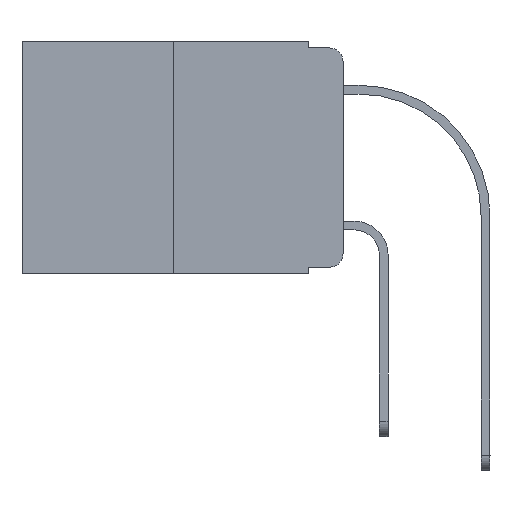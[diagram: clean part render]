
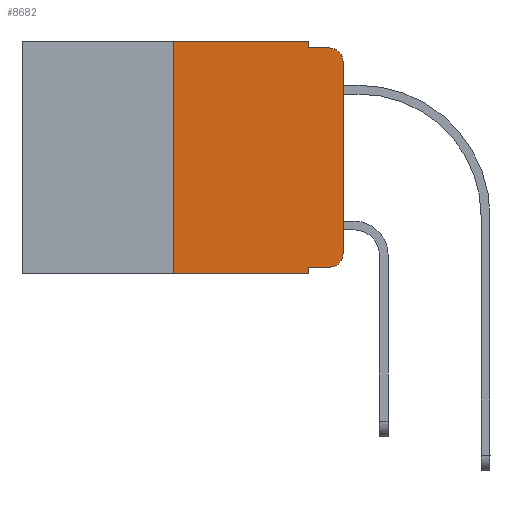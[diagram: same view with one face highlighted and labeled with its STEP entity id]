
A CAD part, left-side view. The second image highlights one B-rep face of the part: STEP entity #8682.
In plain terms, the highlighted planar face has unit normal (-1, 0, 0).
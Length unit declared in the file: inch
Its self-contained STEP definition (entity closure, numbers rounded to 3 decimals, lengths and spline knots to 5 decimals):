
#50 = AXIS2_PLACEMENT_3D ( 'NONE', #10826, #472, #3519 ) ;
#267 = CARTESIAN_POINT ( 'NONE',  ( 0., 0.051, -0.333 ) ) ;
#313 = LINE ( 'NONE', #8908, #887 ) ;
#472 = DIRECTION ( 'NONE',  ( -1., 0., 0. ) ) ;
#727 = ORIENTED_EDGE ( 'NONE', *, *, #12089, .T. ) ;
#887 = VECTOR ( 'NONE', #5989, 39.37008 ) ;
#927 = VERTEX_POINT ( 'NONE', #12649 ) ;
#1011 = DIRECTION ( 'NONE',  ( 0., -1., 0. ) ) ;
#1066 = EDGE_LOOP ( 'NONE', ( #11699, #17623, #16235, #14719, #14676, #9223, #13235, #10024, #4918, #727 ) ) ;
#1161 = DIRECTION ( 'NONE',  ( 0., 0., 1. ) ) ;
#1207 = CIRCLE ( 'NONE', #12118, 0.02 ) ;
#1304 = VERTEX_POINT ( 'NONE', #11146 ) ;
#1893 = VERTEX_POINT ( 'NONE', #14709 ) ;
#2257 = EDGE_CURVE ( 'NONE', #16215, #1304, #1207, .T. ) ;
#2621 = LINE ( 'NONE', #8669, #13465 ) ;
#2675 = LINE ( 'NONE', #18884, #6935 ) ;
#2961 = CARTESIAN_POINT ( 'NONE',  ( 0., 0.473, 0. ) ) ;
#3015 = LINE ( 'NONE', #267, #4621 ) ;
#3328 = DIRECTION ( 'NONE',  ( 0., 0., -1. ) ) ;
#3519 = DIRECTION ( 'NONE',  ( 0., 0., -1. ) ) ;
#3667 = EDGE_CURVE ( 'NONE', #16139, #12094, #17887, .T. ) ;
#4338 = CARTESIAN_POINT ( 'NONE',  ( 0., 0., 0. ) ) ;
#4597 = CARTESIAN_POINT ( 'NONE',  ( 0., 0.02, -0.03 ) ) ;
#4621 = VECTOR ( 'NONE', #16482, 39.37008 ) ;
#4918 = ORIENTED_EDGE ( 'NONE', *, *, #7769, .T. ) ;
#5019 = VERTEX_POINT ( 'NONE', #17820 ) ;
#5074 = CARTESIAN_POINT ( 'NONE',  ( 0., 0.051, 0. ) ) ;
#5329 = VECTOR ( 'NONE', #7359, 39.37008 ) ;
#5377 = CARTESIAN_POINT ( 'NONE',  ( 0., 0.25, 0. ) ) ;
#5652 = DIRECTION ( 'NONE',  ( 0., -1., 0. ) ) ;
#5989 = DIRECTION ( 'NONE',  ( 0., -1., 0. ) ) ;
#6250 = DIRECTION ( 'NONE',  ( 0., 0., -1. ) ) ;
#6935 = VECTOR ( 'NONE', #1011, 39.37008 ) ;
#7359 = DIRECTION ( 'NONE',  ( 0., 0., 1. ) ) ;
#7623 = DIRECTION ( 'NONE',  ( -1., 0., 0. ) ) ;
#7769 = EDGE_CURVE ( 'NONE', #17318, #11249, #3015, .T. ) ;
#8669 = CARTESIAN_POINT ( 'NONE',  ( 0., 0.473, 0. ) ) ;
#8682 = ADVANCED_FACE ( 'NONE', ( #17999 ), #16243, .F. ) ;
#8725 = EDGE_CURVE ( 'NONE', #12094, #1304, #313, .T. ) ;
#8908 = CARTESIAN_POINT ( 'NONE',  ( 0., 0.051, -0.01 ) ) ;
#9108 = DIRECTION ( 'NONE',  ( 0., 0., -1. ) ) ;
#9223 = ORIENTED_EDGE ( 'NONE', *, *, #10721, .F. ) ;
#9567 = LINE ( 'NONE', #5074, #11299 ) ;
#9822 = VERTEX_POINT ( 'NONE', #14780 ) ;
#10024 = ORIENTED_EDGE ( 'NONE', *, *, #12182, .F. ) ;
#10446 = DIRECTION ( 'NONE',  ( 0., 0., -1. ) ) ;
#10721 = EDGE_CURVE ( 'NONE', #9822, #1893, #14545, .T. ) ;
#10826 = CARTESIAN_POINT ( 'NONE',  ( 0., 0.02, -0.313 ) ) ;
#11093 = CARTESIAN_POINT ( 'NONE',  ( 0., 0., -0.03 ) ) ;
#11146 = CARTESIAN_POINT ( 'NONE',  ( 0., 0.02, -0.01 ) ) ;
#11179 = AXIS2_PLACEMENT_3D ( 'NONE', #2961, #11851, #9108 ) ;
#11249 = VERTEX_POINT ( 'NONE', #18303 ) ;
#11299 = VECTOR ( 'NONE', #6250, 39.37008 ) ;
#11387 = EDGE_CURVE ( 'NONE', #9822, #927, #2675, .T. ) ;
#11699 = ORIENTED_EDGE ( 'NONE', *, *, #16464, .T. ) ;
#11851 = DIRECTION ( 'NONE',  ( 1., 0., 0. ) ) ;
#12089 = EDGE_CURVE ( 'NONE', #11249, #5019, #14110, .T. ) ;
#12094 = VERTEX_POINT ( 'NONE', #15529 ) ;
#12118 = AXIS2_PLACEMENT_3D ( 'NONE', #4597, #7623, #3328 ) ;
#12182 = EDGE_CURVE ( 'NONE', #17318, #927, #9567, .T. ) ;
#12361 = CARTESIAN_POINT ( 'NONE',  ( 0., 0.051, 0. ) ) ;
#12649 = CARTESIAN_POINT ( 'NONE',  ( 0., 0.051, -0.343 ) ) ;
#13235 = ORIENTED_EDGE ( 'NONE', *, *, #11387, .T. ) ;
#13437 = LINE ( 'NONE', #4338, #5329 ) ;
#13465 = VECTOR ( 'NONE', #5652, 39.37008 ) ;
#14110 = CIRCLE ( 'NONE', #50, 0.02 ) ;
#14545 = LINE ( 'NONE', #5377, #15114 ) ;
#14638 = CARTESIAN_POINT ( 'NONE',  ( 0., 0.051, -0.333 ) ) ;
#14676 = ORIENTED_EDGE ( 'NONE', *, *, #17266, .F. ) ;
#14709 = CARTESIAN_POINT ( 'NONE',  ( 0., 0.25, 0. ) ) ;
#14719 = ORIENTED_EDGE ( 'NONE', *, *, #3667, .F. ) ;
#14780 = CARTESIAN_POINT ( 'NONE',  ( 0., 0.25, -0.343 ) ) ;
#15114 = VECTOR ( 'NONE', #1161, 39.37008 ) ;
#15245 = VECTOR ( 'NONE', #10446, 39.37008 ) ;
#15529 = CARTESIAN_POINT ( 'NONE',  ( 0., 0.051, -0.01 ) ) ;
#16139 = VERTEX_POINT ( 'NONE', #12361 ) ;
#16215 = VERTEX_POINT ( 'NONE', #11093 ) ;
#16235 = ORIENTED_EDGE ( 'NONE', *, *, #8725, .F. ) ;
#16243 = PLANE ( 'NONE',  #11179 ) ;
#16464 = EDGE_CURVE ( 'NONE', #5019, #16215, #13437, .T. ) ;
#16482 = DIRECTION ( 'NONE',  ( 0., -1., 0. ) ) ;
#17266 = EDGE_CURVE ( 'NONE', #1893, #16139, #2621, .T. ) ;
#17318 = VERTEX_POINT ( 'NONE', #14638 ) ;
#17623 = ORIENTED_EDGE ( 'NONE', *, *, #2257, .T. ) ;
#17820 = CARTESIAN_POINT ( 'NONE',  ( 0., 0., -0.313 ) ) ;
#17887 = LINE ( 'NONE', #19067, #15245 ) ;
#17999 = FACE_OUTER_BOUND ( 'NONE', #1066, .T. ) ;
#18303 = CARTESIAN_POINT ( 'NONE',  ( 0., 0.02, -0.333 ) ) ;
#18884 = CARTESIAN_POINT ( 'NONE',  ( 0., 0.473, -0.343 ) ) ;
#19067 = CARTESIAN_POINT ( 'NONE',  ( 0., 0.051, 0. ) ) ;
